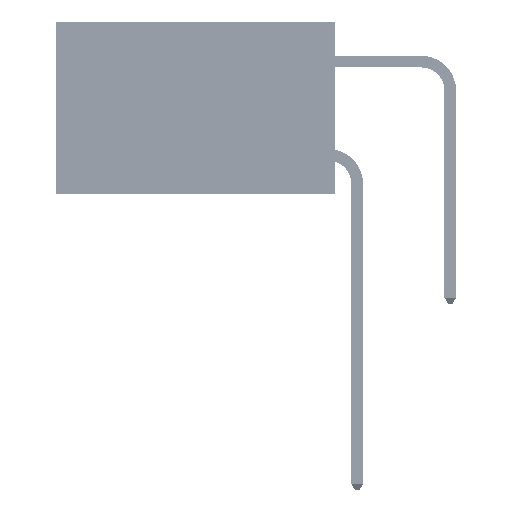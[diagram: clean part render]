
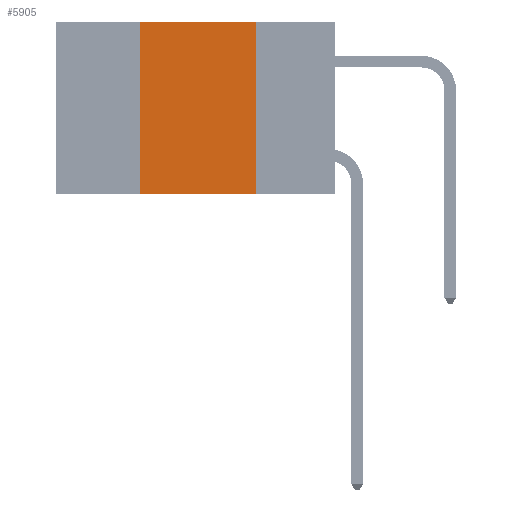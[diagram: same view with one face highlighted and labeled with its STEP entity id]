
A CAD part, left-side view. The second image highlights one B-rep face of the part: STEP entity #5905.
In plain terms, the highlighted planar face has unit normal (-1, 0, 0).
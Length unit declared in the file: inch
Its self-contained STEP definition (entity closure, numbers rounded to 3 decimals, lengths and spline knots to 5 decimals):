
#206 = DIRECTION ( 'NONE',  ( 1., 0., 0. ) ) ;
#1449 = DIRECTION ( 'NONE',  ( 0., -1., 0. ) ) ;
#2869 = EDGE_CURVE ( 'NONE', #24345, #13192, #26624, .T. ) ;
#5905 = ADVANCED_FACE ( 'NONE', ( #39548 ), #27711, .F. ) ;
#6323 = VERTEX_POINT ( 'NONE', #24721 ) ;
#7665 = AXIS2_PLACEMENT_3D ( 'NONE', #24595, #206, #24102 ) ;
#8453 = EDGE_CURVE ( 'NONE', #13192, #6323, #38536, .T. ) ;
#9660 = CARTESIAN_POINT ( 'NONE',  ( 0., 0.6, -0.37 ) ) ;
#12026 = DIRECTION ( 'NONE',  ( 0., 0., -1. ) ) ;
#13192 = VERTEX_POINT ( 'NONE', #46367 ) ;
#13329 = LINE ( 'NONE', #21546, #17622 ) ;
#16688 = DIRECTION ( 'NONE',  ( 0., 0., 1. ) ) ;
#17622 = VECTOR ( 'NONE', #16688, 39.37008 ) ;
#18148 = CARTESIAN_POINT ( 'NONE',  ( 0., 0.6, 0. ) ) ;
#21490 = ORIENTED_EDGE ( 'NONE', *, *, #37947, .F. ) ;
#21546 = CARTESIAN_POINT ( 'NONE',  ( 0., 0.42, 0. ) ) ;
#24102 = DIRECTION ( 'NONE',  ( 0., 0., -1. ) ) ;
#24213 = CARTESIAN_POINT ( 'NONE',  ( 0., 0.42, -0.37 ) ) ;
#24345 = VERTEX_POINT ( 'NONE', #29688 ) ;
#24595 = CARTESIAN_POINT ( 'NONE',  ( 0., 0.6, 0. ) ) ;
#24721 = CARTESIAN_POINT ( 'NONE',  ( 0., 0.17, -0.37 ) ) ;
#26361 = VERTEX_POINT ( 'NONE', #24213 ) ;
#26624 = LINE ( 'NONE', #18148, #45850 ) ;
#26971 = ORIENTED_EDGE ( 'NONE', *, *, #8453, .F. ) ;
#27474 = CARTESIAN_POINT ( 'NONE',  ( 0., 0.17, 0. ) ) ;
#27711 = PLANE ( 'NONE',  #7665 ) ;
#29688 = CARTESIAN_POINT ( 'NONE',  ( 0., 0.42, 0. ) ) ;
#32938 = VECTOR ( 'NONE', #1449, 39.37008 ) ;
#36707 = ORIENTED_EDGE ( 'NONE', *, *, #2869, .F. ) ;
#37947 = EDGE_CURVE ( 'NONE', #26361, #24345, #13329, .T. ) ;
#38536 = LINE ( 'NONE', #27474, #41246 ) ;
#39548 = FACE_OUTER_BOUND ( 'NONE', #44133, .T. ) ;
#40214 = ORIENTED_EDGE ( 'NONE', *, *, #47427, .T. ) ;
#41246 = VECTOR ( 'NONE', #12026, 39.37008 ) ;
#41546 = LINE ( 'NONE', #9660, #32938 ) ;
#42330 = DIRECTION ( 'NONE',  ( 0., -1., 0. ) ) ;
#44133 = EDGE_LOOP ( 'NONE', ( #26971, #36707, #21490, #40214 ) ) ;
#45850 = VECTOR ( 'NONE', #42330, 39.37008 ) ;
#46367 = CARTESIAN_POINT ( 'NONE',  ( 0., 0.17, 0. ) ) ;
#47427 = EDGE_CURVE ( 'NONE', #26361, #6323, #41546, .T. ) ;
